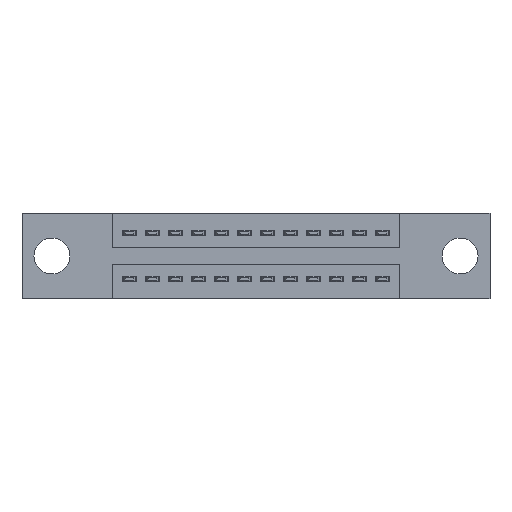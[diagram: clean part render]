
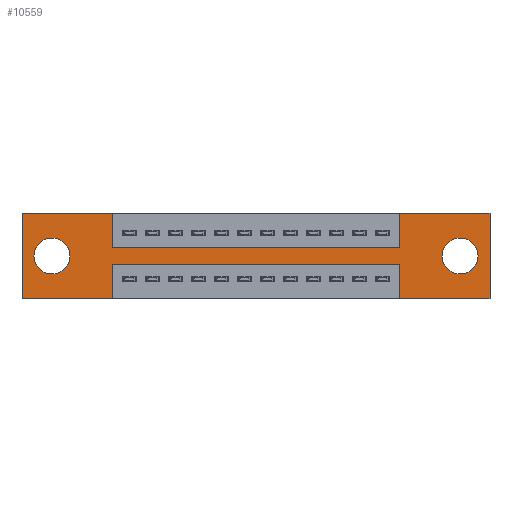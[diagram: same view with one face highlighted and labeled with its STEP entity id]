
A CAD part, front view. The second image highlights one B-rep face of the part: STEP entity #10559.
In plain terms, the highlighted planar face has unit normal (0, -1, 0).
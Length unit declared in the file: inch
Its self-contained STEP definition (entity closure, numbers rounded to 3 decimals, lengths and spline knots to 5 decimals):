
#7 = CARTESIAN_POINT ( 'NONE',  ( 0., 0., 0. ) ) ;
#17 = AXIS2_PLACEMENT_3D ( 'NONE', #9547, #3303, #10570 ) ;
#154 = DIRECTION ( 'NONE',  ( 1., 0., 0. ) ) ;
#324 = EDGE_CURVE ( 'NONE', #9591, #11641, #6727, .T. ) ;
#446 = CIRCLE ( 'NONE', #12091, 0.078 ) ;
#560 = EDGE_LOOP ( 'NONE', ( #1815, #1827, #1831, #1955, #1964, #2005, #2072, #2099, #2165, #2306, #2400, #2444 ) ) ;
#666 = VERTEX_POINT ( 'NONE', #4082 ) ;
#750 = FACE_BOUND ( 'NONE', #6367, .T. ) ;
#822 = EDGE_CURVE ( 'NONE', #6348, #6557, #9691, .T. ) ;
#828 = DIRECTION ( 'NONE',  ( 0., 1., 0. ) ) ;
#884 = DIRECTION ( 'NONE',  ( 0., 1., 0. ) ) ;
#993 = EDGE_CURVE ( 'NONE', #11641, #1384, #7391, .T. ) ;
#1001 = LINE ( 'NONE', #7751, #3746 ) ;
#1036 = AXIS2_PLACEMENT_3D ( 'NONE', #1310, #7113, #1319 ) ;
#1037 = CARTESIAN_POINT ( 'NONE',  ( 0.3925, 0., 0. ) ) ;
#1060 = CIRCLE ( 'NONE', #1036, 0.078 ) ;
#1119 = CARTESIAN_POINT ( 'NONE',  ( 0., 0., -0.37 ) ) ;
#1191 = ORIENTED_EDGE ( 'NONE', *, *, #10439, .T. ) ;
#1217 = ORIENTED_EDGE ( 'NONE', *, *, #10649, .T. ) ;
#1284 = VERTEX_POINT ( 'NONE', #6235 ) ;
#1310 = CARTESIAN_POINT ( 'NONE',  ( 0.13, 0., -0.185 ) ) ;
#1319 = DIRECTION ( 'NONE',  ( 0., 0., 1. ) ) ;
#1384 = VERTEX_POINT ( 'NONE', #11600 ) ;
#1485 = ORIENTED_EDGE ( 'NONE', *, *, #2182, .T. ) ;
#1777 = ORIENTED_EDGE ( 'NONE', *, *, #5104, .T. ) ;
#1815 = ORIENTED_EDGE ( 'NONE', *, *, #324, .F. ) ;
#1827 = ORIENTED_EDGE ( 'NONE', *, *, #6839, .F. ) ;
#1831 = ORIENTED_EDGE ( 'NONE', *, *, #3414, .F. ) ;
#1848 = EDGE_CURVE ( 'NONE', #1284, #4890, #2826, .T. ) ;
#1955 = ORIENTED_EDGE ( 'NONE', *, *, #4229, .F. ) ;
#1964 = ORIENTED_EDGE ( 'NONE', *, *, #7405, .F. ) ;
#2005 = ORIENTED_EDGE ( 'NONE', *, *, #11490, .F. ) ;
#2072 = ORIENTED_EDGE ( 'NONE', *, *, #1848, .F. ) ;
#2099 = ORIENTED_EDGE ( 'NONE', *, *, #4018, .F. ) ;
#2139 = CARTESIAN_POINT ( 'NONE',  ( 0.13, 0., -0.263 ) ) ;
#2151 = DIRECTION ( 'NONE',  ( 0., -1., 0. ) ) ;
#2165 = ORIENTED_EDGE ( 'NONE', *, *, #4339, .F. ) ;
#2182 = EDGE_CURVE ( 'NONE', #11567, #9283, #1060, .T. ) ;
#2194 = LINE ( 'NONE', #8670, #7709 ) ;
#2291 = DIRECTION ( 'NONE',  ( 1., 0., 0. ) ) ;
#2306 = ORIENTED_EDGE ( 'NONE', *, *, #822, .F. ) ;
#2388 = AXIS2_PLACEMENT_3D ( 'NONE', #7067, #884, #8163 ) ;
#2400 = ORIENTED_EDGE ( 'NONE', *, *, #9287, .F. ) ;
#2405 = DIRECTION ( 'NONE',  ( 0., 0., -1. ) ) ;
#2411 = VECTOR ( 'NONE', #4967, 39.37008 ) ;
#2444 = ORIENTED_EDGE ( 'NONE', *, *, #993, .F. ) ;
#2826 = LINE ( 'NONE', #5159, #4964 ) ;
#2980 = CARTESIAN_POINT ( 'NONE',  ( 1.6425, 0., -0.22 ) ) ;
#3144 = VECTOR ( 'NONE', #154, 39.37008 ) ;
#3255 = VERTEX_POINT ( 'NONE', #2980 ) ;
#3303 = DIRECTION ( 'NONE',  ( 0., 1., 0. ) ) ;
#3414 = EDGE_CURVE ( 'NONE', #11899, #3255, #10579, .T. ) ;
#3487 = FACE_OUTER_BOUND ( 'NONE', #560, .T. ) ;
#3554 = DIRECTION ( 'NONE',  ( -1., 0., 0. ) ) ;
#3746 = VECTOR ( 'NONE', #7725, 39.37008 ) ;
#3872 = VERTEX_POINT ( 'NONE', #8860 ) ;
#4018 = EDGE_CURVE ( 'NONE', #4281, #1284, #1001, .T. ) ;
#4053 = DIRECTION ( 'NONE',  ( 0., 0., -1. ) ) ;
#4082 = CARTESIAN_POINT ( 'NONE',  ( 1.905, 0., -0.107 ) ) ;
#4137 = CARTESIAN_POINT ( 'NONE',  ( 0.3925, 0., 0. ) ) ;
#4229 = EDGE_CURVE ( 'NONE', #3872, #11899, #10685, .T. ) ;
#4281 = VERTEX_POINT ( 'NONE', #4700 ) ;
#4339 = EDGE_CURVE ( 'NONE', #6557, #4281, #12082, .T. ) ;
#4382 = LINE ( 'NONE', #7, #10726 ) ;
#4688 = VECTOR ( 'NONE', #7147, 39.37008 ) ;
#4691 = CARTESIAN_POINT ( 'NONE',  ( 1.6425, 0., 0. ) ) ;
#4700 = CARTESIAN_POINT ( 'NONE',  ( 0.3925, 0., -0.15 ) ) ;
#4890 = VERTEX_POINT ( 'NONE', #4691 ) ;
#4964 = VECTOR ( 'NONE', #7063, 39.37008 ) ;
#4967 = DIRECTION ( 'NONE',  ( -1., 0., 0. ) ) ;
#4994 = CARTESIAN_POINT ( 'NONE',  ( 1.6425, 0., -0.37 ) ) ;
#5104 = EDGE_CURVE ( 'NONE', #9283, #11567, #446, .T. ) ;
#5159 = CARTESIAN_POINT ( 'NONE',  ( 1.6425, 0., 0. ) ) ;
#5299 = CIRCLE ( 'NONE', #17, 0.078 ) ;
#5436 = CARTESIAN_POINT ( 'NONE',  ( 0., 0., -0.37 ) ) ;
#5901 = CARTESIAN_POINT ( 'NONE',  ( 1.905, 0., -0.263 ) ) ;
#6235 = CARTESIAN_POINT ( 'NONE',  ( 1.6425, 0., -0.15 ) ) ;
#6268 = FACE_BOUND ( 'NONE', #10300, .T. ) ;
#6348 = VERTEX_POINT ( 'NONE', #12031 ) ;
#6367 = EDGE_LOOP ( 'NONE', ( #1191, #1217 ) ) ;
#6557 = VERTEX_POINT ( 'NONE', #1037 ) ;
#6727 = LINE ( 'NONE', #9589, #4688 ) ;
#6839 = EDGE_CURVE ( 'NONE', #3255, #9591, #9077, .T. ) ;
#6901 = VECTOR ( 'NONE', #2291, 39.37008 ) ;
#7025 = CARTESIAN_POINT ( 'NONE',  ( 0.13, 0., -0.185 ) ) ;
#7063 = DIRECTION ( 'NONE',  ( 0., 0., 1. ) ) ;
#7067 = CARTESIAN_POINT ( 'NONE',  ( 1.905, 0., -0.185 ) ) ;
#7104 = CIRCLE ( 'NONE', #2388, 0.078 ) ;
#7113 = DIRECTION ( 'NONE',  ( 0., 1., 0. ) ) ;
#7147 = DIRECTION ( 'NONE',  ( 0., 0., -1. ) ) ;
#7391 = LINE ( 'NONE', #7990, #10489 ) ;
#7405 = EDGE_CURVE ( 'NONE', #10554, #3872, #2194, .T. ) ;
#7709 = VECTOR ( 'NONE', #2405, 39.37008 ) ;
#7725 = DIRECTION ( 'NONE',  ( 1., 0., 0. ) ) ;
#7751 = CARTESIAN_POINT ( 'NONE',  ( 0.3925, 0., -0.15 ) ) ;
#7830 = VECTOR ( 'NONE', #12378, 39.37008 ) ;
#7990 = CARTESIAN_POINT ( 'NONE',  ( 0., 0., -0.37 ) ) ;
#8110 = DIRECTION ( 'NONE',  ( 0., 0., 1. ) ) ;
#8163 = DIRECTION ( 'NONE',  ( 0., 0., -1. ) ) ;
#8347 = CARTESIAN_POINT ( 'NONE',  ( 2.035, 0., 0. ) ) ;
#8400 = PLANE ( 'NONE',  #10728 ) ;
#8670 = CARTESIAN_POINT ( 'NONE',  ( 2.035, 0., 0. ) ) ;
#8747 = CARTESIAN_POINT ( 'NONE',  ( 0.3925, 0., -0.37 ) ) ;
#8860 = CARTESIAN_POINT ( 'NONE',  ( 2.035, 0., -0.37 ) ) ;
#8874 = CARTESIAN_POINT ( 'NONE',  ( 0.3925, 0., -0.22 ) ) ;
#9077 = LINE ( 'NONE', #8874, #11437 ) ;
#9283 = VERTEX_POINT ( 'NONE', #2139 ) ;
#9287 = EDGE_CURVE ( 'NONE', #1384, #6348, #4382, .T. ) ;
#9434 = DIRECTION ( 'NONE',  ( 0., 0., -1. ) ) ;
#9547 = CARTESIAN_POINT ( 'NONE',  ( 1.905, 0., -0.185 ) ) ;
#9589 = CARTESIAN_POINT ( 'NONE',  ( 0.3925, 0., -0.37 ) ) ;
#9591 = VERTEX_POINT ( 'NONE', #10966 ) ;
#9691 = LINE ( 'NONE', #11253, #6901 ) ;
#10300 = EDGE_LOOP ( 'NONE', ( #1485, #1777 ) ) ;
#10430 = DIRECTION ( 'NONE',  ( 0., 0., 1. ) ) ;
#10439 = EDGE_CURVE ( 'NONE', #666, #10830, #7104, .T. ) ;
#10489 = VECTOR ( 'NONE', #3554, 39.37008 ) ;
#10554 = VERTEX_POINT ( 'NONE', #8347 ) ;
#10559 = ADVANCED_FACE ( 'NONE', ( #750, #6268, #3487 ), #8400, .T. ) ;
#10570 = DIRECTION ( 'NONE',  ( 0., 0., -1. ) ) ;
#10579 = LINE ( 'NONE', #12455, #7830 ) ;
#10649 = EDGE_CURVE ( 'NONE', #10830, #666, #5299, .T. ) ;
#10685 = LINE ( 'NONE', #5436, #2411 ) ;
#10726 = VECTOR ( 'NONE', #10430, 39.37008 ) ;
#10728 = AXIS2_PLACEMENT_3D ( 'NONE', #1119, #2151, #9434 ) ;
#10830 = VERTEX_POINT ( 'NONE', #5901 ) ;
#10904 = DIRECTION ( 'NONE',  ( -1., 0., 0. ) ) ;
#10966 = CARTESIAN_POINT ( 'NONE',  ( 0.3925, 0., -0.22 ) ) ;
#11253 = CARTESIAN_POINT ( 'NONE',  ( 0., 0., 0. ) ) ;
#11422 = LINE ( 'NONE', #11540, #3144 ) ;
#11437 = VECTOR ( 'NONE', #10904, 39.37008 ) ;
#11490 = EDGE_CURVE ( 'NONE', #4890, #10554, #11422, .T. ) ;
#11540 = CARTESIAN_POINT ( 'NONE',  ( 0., 0., 0. ) ) ;
#11567 = VERTEX_POINT ( 'NONE', #11666 ) ;
#11600 = CARTESIAN_POINT ( 'NONE',  ( 0., 0., -0.37 ) ) ;
#11641 = VERTEX_POINT ( 'NONE', #8747 ) ;
#11666 = CARTESIAN_POINT ( 'NONE',  ( 0.13, 0., -0.107 ) ) ;
#11793 = VECTOR ( 'NONE', #4053, 39.37008 ) ;
#11899 = VERTEX_POINT ( 'NONE', #4994 ) ;
#12031 = CARTESIAN_POINT ( 'NONE',  ( 0., 0., 0. ) ) ;
#12082 = LINE ( 'NONE', #4137, #11793 ) ;
#12091 = AXIS2_PLACEMENT_3D ( 'NONE', #7025, #828, #8110 ) ;
#12378 = DIRECTION ( 'NONE',  ( 0., 0., 1. ) ) ;
#12455 = CARTESIAN_POINT ( 'NONE',  ( 1.6425, 0., -0.37 ) ) ;
